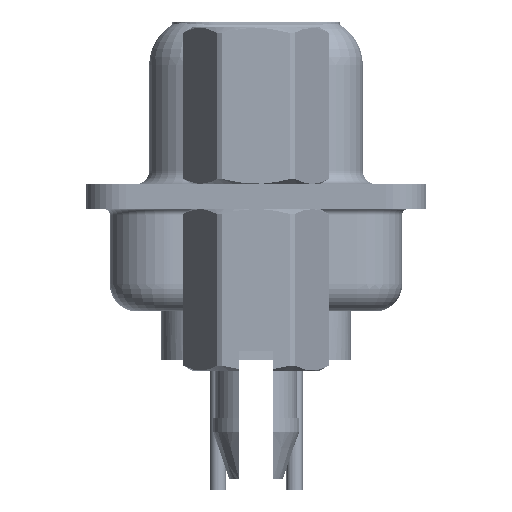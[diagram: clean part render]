
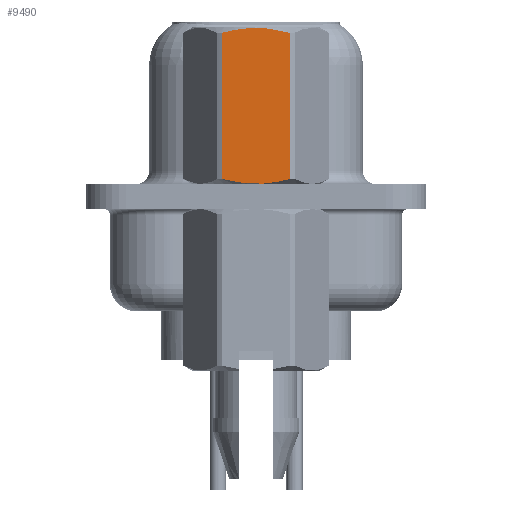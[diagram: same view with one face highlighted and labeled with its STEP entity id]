
A CAD part, left-side view. The second image highlights one B-rep face of the part: STEP entity #9490.
In plain terms, the highlighted planar face has unit normal (-1, 0, 0).
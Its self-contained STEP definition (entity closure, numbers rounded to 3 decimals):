
#675 = CARTESIAN_POINT ( 'NONE',  ( -2.381, -1.273, 3.792 ) ) ;
#1095 = ORIENTED_EDGE ( 'NONE', *, *, #3800, .T. ) ;
#1172 = CARTESIAN_POINT ( 'NONE',  ( -2.381, -1.066, 0.596 ) ) ;
#1247 = LINE ( 'NONE', #675, #12450 ) ;
#2642 = CARTESIAN_POINT ( 'NONE',  ( -2.381, 1.065, 6.104 ) ) ;
#3800 = EDGE_CURVE ( 'NONE', #10416, #4317, #24633, .T. ) ;
#3890 = CARTESIAN_POINT ( 'NONE',  ( -2.381, -0.215, 0.468 ) ) ;
#4079 = CARTESIAN_POINT ( 'NONE',  ( -2.381, 1.065, 0.596 ) ) ;
#4317 = VERTEX_POINT ( 'NONE', #8230 ) ;
#4376 = ORIENTED_EDGE ( 'NONE', *, *, #20286, .T. ) ;
#4680 = VERTEX_POINT ( 'NONE', #28989 ) ;
#4838 = DIRECTION ( 'NONE',  ( 0., -1., 0. ) ) ;
#5022 = ORIENTED_EDGE ( 'NONE', *, *, #37832, .T. ) ;
#5394 = CARTESIAN_POINT ( 'NONE',  ( -2.381, 0.428, 6.215 ) ) ;
#5496 = VECTOR ( 'NONE', #17922, 1000. ) ;
#7032 = CARTESIAN_POINT ( 'NONE',  ( -2.381, -1.273, 0.652 ) ) ;
#7792 = PLANE ( 'NONE',  #16216 ) ;
#7969 = CARTESIAN_POINT ( 'NONE',  ( -2.381, 1.375, -3.75 ) ) ;
#8230 = CARTESIAN_POINT ( 'NONE',  ( -2.381, 1.273, 0.652 ) ) ;
#9490 = ADVANCED_FACE ( 'NONE', ( #16643 ), #7792, .T. ) ;
#9977 = CARTESIAN_POINT ( 'NONE',  ( -2.381, -0.432, 0.485 ) ) ;
#10416 = VERTEX_POINT ( 'NONE', #18015 ) ;
#11484 = CARTESIAN_POINT ( 'NONE',  ( -2.381, -0.432, 6.215 ) ) ;
#12450 = VECTOR ( 'NONE', #21662, 1000. ) ;
#16216 = AXIS2_PLACEMENT_3D ( 'NONE', #7969, #31715, #4838 ) ;
#16643 = FACE_OUTER_BOUND ( 'NONE', #28749, .T. ) ;
#16695 = ORIENTED_EDGE ( 'NONE', *, *, #27886, .T. ) ;
#17922 = DIRECTION ( 'NONE',  ( 0., 0., -1. ) ) ;
#18015 = CARTESIAN_POINT ( 'NONE',  ( -2.381, 1.273, 6.048 ) ) ;
#19049 = B_SPLINE_CURVE_WITH_KNOTS ( 'NONE', 3,
 ( #32081, #26399, #38337, #11484, #23069, #35194, #5394, #20907, #2642, #35575 ),
 .UNSPECIFIED., .F., .F.,
 ( 4, 2, 2, 2, 4 ),
 ( 0.001, 0.002, 0.002, 0.003, 0.004 ),
 .UNSPECIFIED. ) ;
#20286 = EDGE_CURVE ( 'NONE', #4317, #4680, #22541, .T. ) ;
#20907 = CARTESIAN_POINT ( 'NONE',  ( -2.381, 0.853, 6.151 ) ) ;
#21662 = DIRECTION ( 'NONE',  ( 0., 0., 1. ) ) ;
#22274 = CARTESIAN_POINT ( 'NONE',  ( -2.381, -1.273, 6.048 ) ) ;
#22541 = B_SPLINE_CURVE_WITH_KNOTS ( 'NONE', 3,
 ( #36639, #4079, #28033, #33898, #30779, #3890, #9977, #30976, #1172, #7032 ),
 .UNSPECIFIED., .F., .F.,
 ( 4, 2, 2, 2, 4 ),
 ( 0.003, 0.003, 0.004, 0.004, 0.005 ),
 .UNSPECIFIED. ) ;
#23069 = CARTESIAN_POINT ( 'NONE',  ( -2.381, -0.215, 6.232 ) ) ;
#24633 = LINE ( 'NONE', #33416, #5496 ) ;
#26399 = CARTESIAN_POINT ( 'NONE',  ( -2.381, -1.066, 6.104 ) ) ;
#27886 = EDGE_CURVE ( 'NONE', #4680, #37996, #1247, .T. ) ;
#28033 = CARTESIAN_POINT ( 'NONE',  ( -2.381, 0.853, 0.549 ) ) ;
#28749 = EDGE_LOOP ( 'NONE', ( #4376, #16695, #5022, #1095 ) ) ;
#28989 = CARTESIAN_POINT ( 'NONE',  ( -2.381, -1.273, 0.652 ) ) ;
#30779 = CARTESIAN_POINT ( 'NONE',  ( -2.381, 0.215, 0.468 ) ) ;
#30976 = CARTESIAN_POINT ( 'NONE',  ( -2.381, -0.858, 0.55 ) ) ;
#31715 = DIRECTION ( 'NONE',  ( -1., 0., 0. ) ) ;
#32081 = CARTESIAN_POINT ( 'NONE',  ( -2.381, -1.273, 6.048 ) ) ;
#33416 = CARTESIAN_POINT ( 'NONE',  ( -2.381, 1.273, 3.792 ) ) ;
#33898 = CARTESIAN_POINT ( 'NONE',  ( -2.381, 0.428, 0.485 ) ) ;
#35194 = CARTESIAN_POINT ( 'NONE',  ( -2.381, 0.215, 6.232 ) ) ;
#35575 = CARTESIAN_POINT ( 'NONE',  ( -2.381, 1.273, 6.048 ) ) ;
#36639 = CARTESIAN_POINT ( 'NONE',  ( -2.381, 1.273, 0.652 ) ) ;
#37832 = EDGE_CURVE ( 'NONE', #37996, #10416, #19049, .T. ) ;
#37996 = VERTEX_POINT ( 'NONE', #22274 ) ;
#38337 = CARTESIAN_POINT ( 'NONE',  ( -2.381, -0.858, 6.15 ) ) ;
